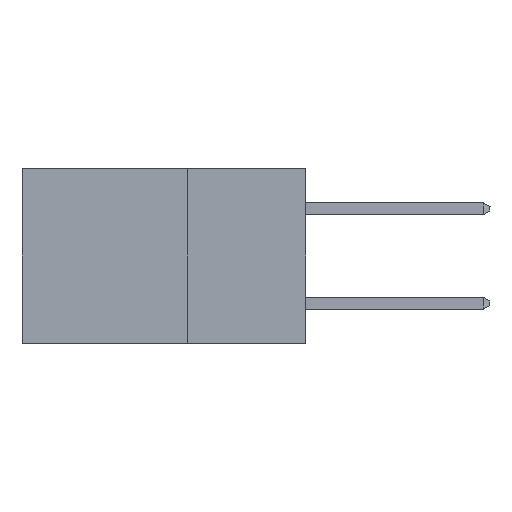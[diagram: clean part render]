
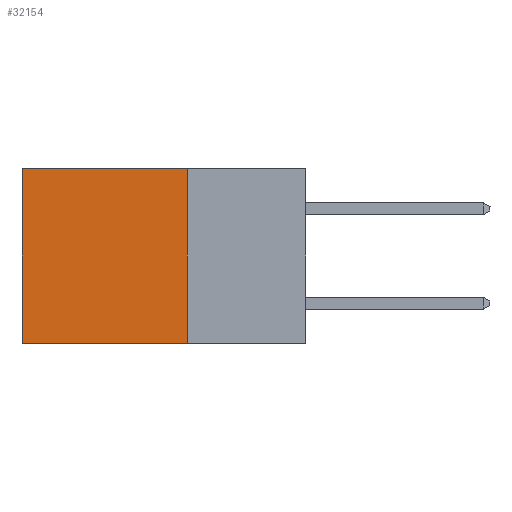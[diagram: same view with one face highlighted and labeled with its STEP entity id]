
A CAD part, left-side view. The second image highlights one B-rep face of the part: STEP entity #32154.
In plain terms, the highlighted planar face has unit normal (-1, 0, 0).
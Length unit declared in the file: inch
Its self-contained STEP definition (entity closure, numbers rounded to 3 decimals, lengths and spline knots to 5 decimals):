
#1106 = VECTOR ( 'NONE', #17231, 39.37008 ) ;
#2572 = EDGE_CURVE ( 'NONE', #9956, #19346, #3656, .T. ) ;
#2893 = CARTESIAN_POINT ( 'NONE',  ( 0.298, 0.6, 0. ) ) ;
#3341 = DIRECTION ( 'NONE',  ( 0., 1., 0. ) ) ;
#3656 = LINE ( 'NONE', #32018, #9791 ) ;
#6570 = CARTESIAN_POINT ( 'NONE',  ( 0.298, 0.25, -0.37 ) ) ;
#6980 = DIRECTION ( 'NONE',  ( 0., 0., -1. ) ) ;
#8747 = AXIS2_PLACEMENT_3D ( 'NONE', #14655, #22463, #6980 ) ;
#9480 = ORIENTED_EDGE ( 'NONE', *, *, #20910, .T. ) ;
#9791 = VECTOR ( 'NONE', #31981, 39.37008 ) ;
#9956 = VERTEX_POINT ( 'NONE', #29749 ) ;
#11182 = LINE ( 'NONE', #6570, #25699 ) ;
#14063 = LINE ( 'NONE', #32461, #1106 ) ;
#14349 = ORIENTED_EDGE ( 'NONE', *, *, #2572, .F. ) ;
#14655 = CARTESIAN_POINT ( 'NONE',  ( 0.298, 0.25, 0. ) ) ;
#17231 = DIRECTION ( 'NONE',  ( 0., 0., -1. ) ) ;
#18860 = CARTESIAN_POINT ( 'NONE',  ( 0.298, 0.25, 0. ) ) ;
#19346 = VERTEX_POINT ( 'NONE', #27296 ) ;
#19441 = CARTESIAN_POINT ( 'NONE',  ( 0.298, 0.6, -0.37 ) ) ;
#19873 = PLANE ( 'NONE',  #8747 ) ;
#20910 = EDGE_CURVE ( 'NONE', #24603, #27511, #14063, .T. ) ;
#22053 = EDGE_CURVE ( 'NONE', #19346, #27511, #11182, .T. ) ;
#22463 = DIRECTION ( 'NONE',  ( 1., 0., 0. ) ) ;
#24603 = VERTEX_POINT ( 'NONE', #2893 ) ;
#24633 = DIRECTION ( 'NONE',  ( 0., 1., 0. ) ) ;
#24714 = EDGE_CURVE ( 'NONE', #9956, #24603, #26313, .T. ) ;
#25699 = VECTOR ( 'NONE', #24633, 39.37008 ) ;
#26313 = LINE ( 'NONE', #18860, #32172 ) ;
#27296 = CARTESIAN_POINT ( 'NONE',  ( 0.298, 0.25, -0.37 ) ) ;
#27511 = VERTEX_POINT ( 'NONE', #19441 ) ;
#27920 = ORIENTED_EDGE ( 'NONE', *, *, #24714, .T. ) ;
#29010 = FACE_OUTER_BOUND ( 'NONE', #32465, .T. ) ;
#29341 = ORIENTED_EDGE ( 'NONE', *, *, #22053, .F. ) ;
#29749 = CARTESIAN_POINT ( 'NONE',  ( 0.298, 0.25, 0. ) ) ;
#31981 = DIRECTION ( 'NONE',  ( 0., 0., -1. ) ) ;
#32018 = CARTESIAN_POINT ( 'NONE',  ( 0.298, 0.25, 0. ) ) ;
#32154 = ADVANCED_FACE ( 'NONE', ( #29010 ), #19873, .F. ) ;
#32172 = VECTOR ( 'NONE', #3341, 39.37008 ) ;
#32461 = CARTESIAN_POINT ( 'NONE',  ( 0.298, 0.6, 0. ) ) ;
#32465 = EDGE_LOOP ( 'NONE', ( #9480, #29341, #14349, #27920 ) ) ;
